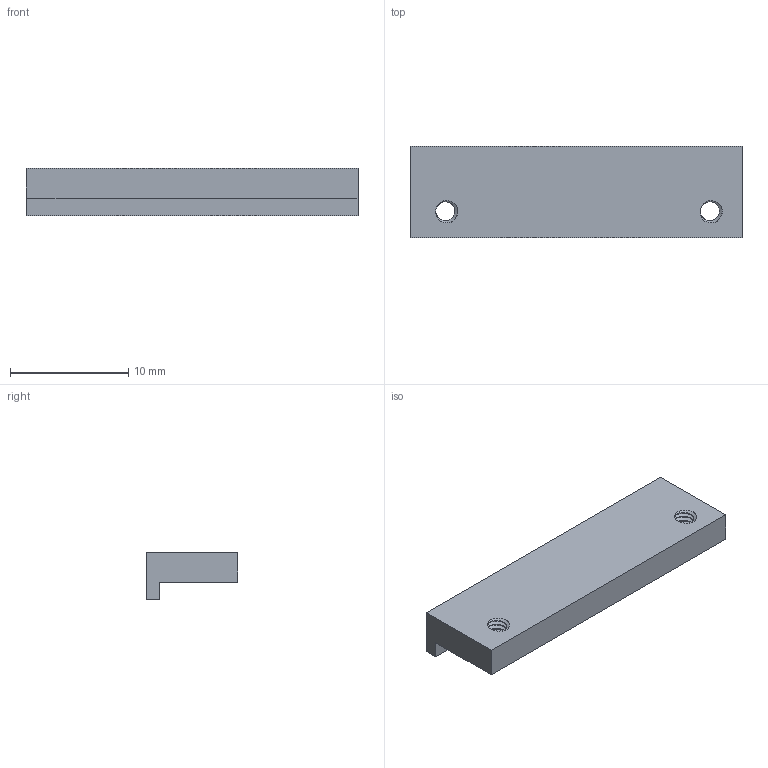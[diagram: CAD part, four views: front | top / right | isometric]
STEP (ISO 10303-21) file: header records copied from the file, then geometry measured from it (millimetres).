
FILE_DESCRIPTION(/* description */ (''),/* implementation_level */ '2;1');
FILE_NAME(/* name */ 'Left Rail Section.stp',/* time_stamp */ '2019-03-17T16:27:31-05:00',/* author */ ('johne'),/* organization */ (''),/* preprocessor_version */ 'ST-DEVELOPER v16.13',/* originating_system */ 'Autodesk Inventor 2018',/* authorisation */ '');
FILE_SCHEMA (('AUTOMOTIVE_DESIGN { 1 0 10303 214 3 1 1 }'));
Length unit declared in the file: millimetre
Products named in the file (1): Component2
Bounding box: 28.11 x 7.78 x 4 mm (x, y, z)
Volume: 588.4 mm3; surface area: 743.1 mm2
Topology: 1 solids, 1 shells, 16 faces, 92 edges, 78 vertices
Faces by surface type: plane 8, cylinder 4, bspline 4
Entity records: 9109 total; most frequent: CARTESIAN_POINT 8449, ORIENTED_EDGE 184, EDGE_CURVE 92, VERTEX_POINT 78, B_SPLINE_CURVE_WITH_KNOTS 64, DIRECTION 64, AXIS2_PLACEMENT_3D 23, EDGE_LOOP 20
